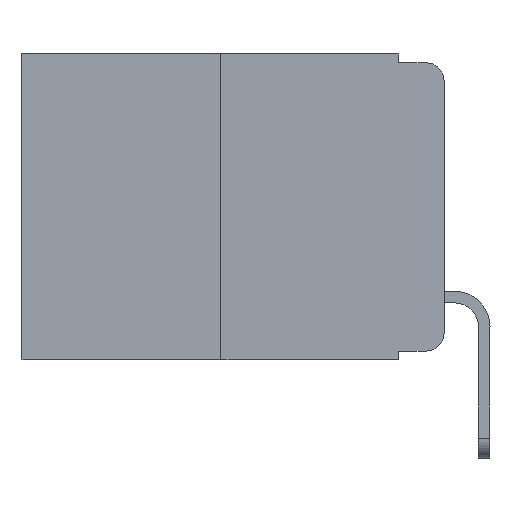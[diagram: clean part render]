
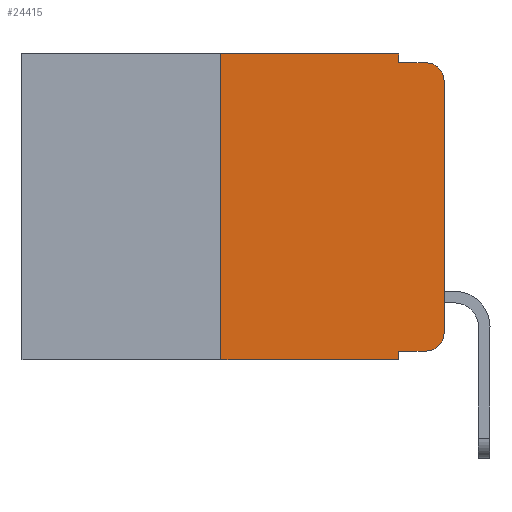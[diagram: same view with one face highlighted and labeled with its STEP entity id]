
A CAD part, left-side view. The second image highlights one B-rep face of the part: STEP entity #24415.
In plain terms, the highlighted planar face has unit normal (-1, 0, 0).
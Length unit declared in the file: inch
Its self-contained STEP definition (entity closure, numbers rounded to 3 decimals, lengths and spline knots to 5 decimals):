
#410 = CARTESIAN_POINT ( 'NONE',  ( 0., 0.051, -0.333 ) ) ;
#1038 = DIRECTION ( 'NONE',  ( 0., 0., -1. ) ) ;
#1065 = DIRECTION ( 'NONE',  ( 0., 0., 1. ) ) ;
#1076 = VERTEX_POINT ( 'NONE', #11095 ) ;
#1240 = VERTEX_POINT ( 'NONE', #3406 ) ;
#1350 = VECTOR ( 'NONE', #5886, 39.37008 ) ;
#1823 = ORIENTED_EDGE ( 'NONE', *, *, #23666, .T. ) ;
#1938 = CARTESIAN_POINT ( 'NONE',  ( 0., 0., 0. ) ) ;
#2460 = CARTESIAN_POINT ( 'NONE',  ( 0., 0.02, -0.03 ) ) ;
#2555 = ORIENTED_EDGE ( 'NONE', *, *, #22327, .T. ) ;
#2686 = CIRCLE ( 'NONE', #9995, 0.02 ) ;
#3148 = DIRECTION ( 'NONE',  ( 0., -1., 0. ) ) ;
#3256 = LINE ( 'NONE', #9683, #24221 ) ;
#3406 = CARTESIAN_POINT ( 'NONE',  ( 0., 0.051, -0.01 ) ) ;
#3485 = VERTEX_POINT ( 'NONE', #410 ) ;
#3536 = LINE ( 'NONE', #7517, #23870 ) ;
#3992 = PLANE ( 'NONE',  #25188 ) ;
#4075 = CARTESIAN_POINT ( 'NONE',  ( 0., 0.051, 0. ) ) ;
#4251 = VERTEX_POINT ( 'NONE', #24146 ) ;
#4360 = VERTEX_POINT ( 'NONE', #15798 ) ;
#4609 = VERTEX_POINT ( 'NONE', #8007 ) ;
#4909 = CARTESIAN_POINT ( 'NONE',  ( 0., 0.051, 0. ) ) ;
#4994 = EDGE_CURVE ( 'NONE', #1076, #4251, #3536, .T. ) ;
#5069 = VERTEX_POINT ( 'NONE', #24082 ) ;
#5886 = DIRECTION ( 'NONE',  ( 0., 0., 1. ) ) ;
#6012 = CARTESIAN_POINT ( 'NONE',  ( 0., 0.473, 0. ) ) ;
#6102 = DIRECTION ( 'NONE',  ( 0., 0., -1. ) ) ;
#6586 = VECTOR ( 'NONE', #1038, 39.37008 ) ;
#6750 = CIRCLE ( 'NONE', #8626, 0.02 ) ;
#6809 = ORIENTED_EDGE ( 'NONE', *, *, #20487, .F. ) ;
#6967 = ORIENTED_EDGE ( 'NONE', *, *, #4994, .T. ) ;
#7184 = EDGE_LOOP ( 'NONE', ( #18536, #10378, #24241, #12224, #13837, #6809, #6967, #20495, #1823, #2555 ) ) ;
#7335 = LINE ( 'NONE', #1938, #1350 ) ;
#7464 = CARTESIAN_POINT ( 'NONE',  ( 0., 0.25, 0. ) ) ;
#7517 = CARTESIAN_POINT ( 'NONE',  ( 0., 0.473, -0.343 ) ) ;
#7679 = DIRECTION ( 'NONE',  ( -1., 0., 0. ) ) ;
#8007 = CARTESIAN_POINT ( 'NONE',  ( 0., 0.02, -0.333 ) ) ;
#8249 = LINE ( 'NONE', #6012, #19079 ) ;
#8626 = AXIS2_PLACEMENT_3D ( 'NONE', #2460, #20733, #14213 ) ;
#9683 = CARTESIAN_POINT ( 'NONE',  ( 0., 0.051, -0.333 ) ) ;
#9717 = DIRECTION ( 'NONE',  ( 0., 0., -1. ) ) ;
#9892 = EDGE_CURVE ( 'NONE', #1240, #5069, #11844, .T. ) ;
#9995 = AXIS2_PLACEMENT_3D ( 'NONE', #23871, #7679, #9717 ) ;
#10078 = DIRECTION ( 'NONE',  ( 1., 0., 0. ) ) ;
#10378 = ORIENTED_EDGE ( 'NONE', *, *, #22634, .T. ) ;
#10402 = LINE ( 'NONE', #4909, #6586 ) ;
#10709 = VECTOR ( 'NONE', #1065, 39.37008 ) ;
#11095 = CARTESIAN_POINT ( 'NONE',  ( 0., 0.25, -0.343 ) ) ;
#11159 = LINE ( 'NONE', #4075, #20723 ) ;
#11428 = EDGE_CURVE ( 'NONE', #21070, #1240, #11159, .T. ) ;
#11698 = CARTESIAN_POINT ( 'NONE',  ( 0., 0.051, -0.01 ) ) ;
#11844 = LINE ( 'NONE', #11698, #23970 ) ;
#12224 = ORIENTED_EDGE ( 'NONE', *, *, #11428, .F. ) ;
#13390 = EDGE_CURVE ( 'NONE', #18418, #4360, #7335, .T. ) ;
#13837 = ORIENTED_EDGE ( 'NONE', *, *, #24383, .F. ) ;
#14213 = DIRECTION ( 'NONE',  ( 0., 0., -1. ) ) ;
#15798 = CARTESIAN_POINT ( 'NONE',  ( 0., 0., -0.03 ) ) ;
#16884 = CARTESIAN_POINT ( 'NONE',  ( 0., 0., -0.313 ) ) ;
#17100 = LINE ( 'NONE', #19426, #10709 ) ;
#18116 = DIRECTION ( 'NONE',  ( 0., -1., 0. ) ) ;
#18210 = VERTEX_POINT ( 'NONE', #7464 ) ;
#18418 = VERTEX_POINT ( 'NONE', #16884 ) ;
#18536 = ORIENTED_EDGE ( 'NONE', *, *, #13390, .T. ) ;
#18754 = FACE_OUTER_BOUND ( 'NONE', #7184, .T. ) ;
#19079 = VECTOR ( 'NONE', #18116, 39.37008 ) ;
#19426 = CARTESIAN_POINT ( 'NONE',  ( 0., 0.25, 0. ) ) ;
#20241 = CARTESIAN_POINT ( 'NONE',  ( 0., 0.473, 0. ) ) ;
#20487 = EDGE_CURVE ( 'NONE', #1076, #18210, #17100, .T. ) ;
#20495 = ORIENTED_EDGE ( 'NONE', *, *, #25193, .F. ) ;
#20723 = VECTOR ( 'NONE', #6102, 39.37008 ) ;
#20733 = DIRECTION ( 'NONE',  ( -1., 0., 0. ) ) ;
#21070 = VERTEX_POINT ( 'NONE', #23207 ) ;
#22327 = EDGE_CURVE ( 'NONE', #4609, #18418, #2686, .T. ) ;
#22634 = EDGE_CURVE ( 'NONE', #4360, #5069, #6750, .T. ) ;
#23207 = CARTESIAN_POINT ( 'NONE',  ( 0., 0.051, 0. ) ) ;
#23666 = EDGE_CURVE ( 'NONE', #3485, #4609, #3256, .T. ) ;
#23870 = VECTOR ( 'NONE', #3148, 39.37008 ) ;
#23871 = CARTESIAN_POINT ( 'NONE',  ( 0., 0.02, -0.313 ) ) ;
#23925 = DIRECTION ( 'NONE',  ( 0., -1., 0. ) ) ;
#23970 = VECTOR ( 'NONE', #24004, 39.37008 ) ;
#24004 = DIRECTION ( 'NONE',  ( 0., -1., 0. ) ) ;
#24082 = CARTESIAN_POINT ( 'NONE',  ( 0., 0.02, -0.01 ) ) ;
#24146 = CARTESIAN_POINT ( 'NONE',  ( 0., 0.051, -0.343 ) ) ;
#24221 = VECTOR ( 'NONE', #23925, 39.37008 ) ;
#24241 = ORIENTED_EDGE ( 'NONE', *, *, #9892, .F. ) ;
#24323 = DIRECTION ( 'NONE',  ( 0., 0., -1. ) ) ;
#24383 = EDGE_CURVE ( 'NONE', #18210, #21070, #8249, .T. ) ;
#24415 = ADVANCED_FACE ( 'NONE', ( #18754 ), #3992, .F. ) ;
#25188 = AXIS2_PLACEMENT_3D ( 'NONE', #20241, #10078, #24323 ) ;
#25193 = EDGE_CURVE ( 'NONE', #3485, #4251, #10402, .T. ) ;
